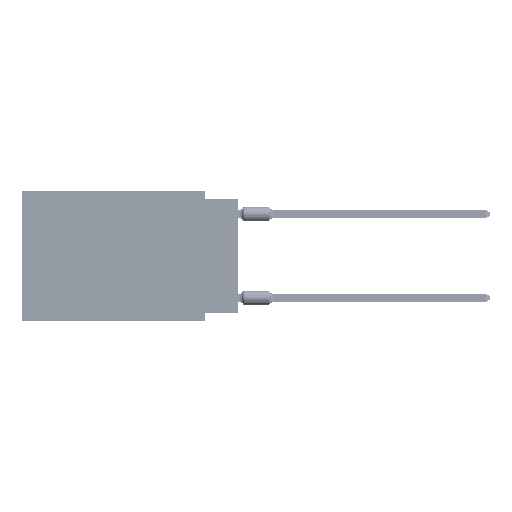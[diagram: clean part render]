
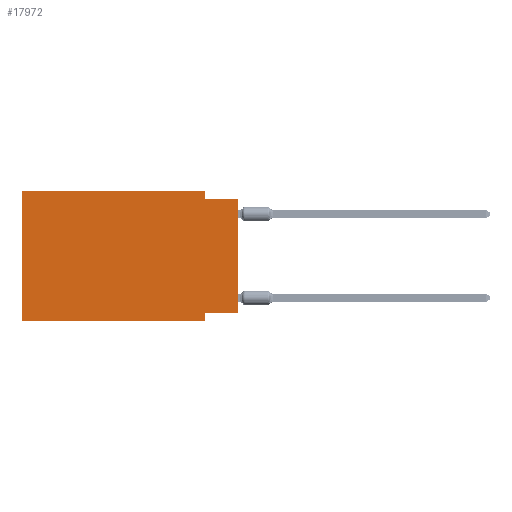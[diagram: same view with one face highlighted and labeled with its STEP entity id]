
A CAD part, left-side view. The second image highlights one B-rep face of the part: STEP entity #17972.
In plain terms, the highlighted planar face has unit normal (-1, 0, 0).
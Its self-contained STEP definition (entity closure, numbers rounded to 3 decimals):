
#256 = CARTESIAN_POINT ( 'NONE',  ( 0., 16.383, 0. ) ) ;
#1149 = VECTOR ( 'NONE', #34853, 1000. ) ;
#2446 = DIRECTION ( 'NONE',  ( 0., 0., -1. ) ) ;
#3097 = FACE_OUTER_BOUND ( 'NONE', #40333, .T. ) ;
#5128 = ORIENTED_EDGE ( 'NONE', *, *, #46602, .F. ) ;
#6071 = VECTOR ( 'NONE', #60997, 1000. ) ;
#8288 = CARTESIAN_POINT ( 'NONE',  ( 0., 2.54, -9.906 ) ) ;
#8918 = EDGE_CURVE ( 'NONE', #62883, #73409, #58326, .T. ) ;
#10476 = DIRECTION ( 'NONE',  ( 0., -1., 0. ) ) ;
#10887 = VECTOR ( 'NONE', #33631, 1000. ) ;
#12662 = VECTOR ( 'NONE', #24476, 1000. ) ;
#12917 = VERTEX_POINT ( 'NONE', #16087 ) ;
#12929 = CARTESIAN_POINT ( 'NONE',  ( 0., 16.383, -9.906 ) ) ;
#14081 = LINE ( 'NONE', #31740, #12662 ) ;
#14102 = CARTESIAN_POINT ( 'NONE',  ( 0., 0., -0.635 ) ) ;
#16087 = CARTESIAN_POINT ( 'NONE',  ( 0., 2.54, -9.906 ) ) ;
#16154 = ORIENTED_EDGE ( 'NONE', *, *, #8918, .F. ) ;
#16762 = EDGE_CURVE ( 'NONE', #73409, #66488, #39295, .T. ) ;
#17756 = CARTESIAN_POINT ( 'NONE',  ( 0., 2.54, -9.271 ) ) ;
#17972 = ADVANCED_FACE ( 'NONE', ( #3097 ), #67305, .F. ) ;
#20250 = CARTESIAN_POINT ( 'NONE',  ( 0., 0., -0.635 ) ) ;
#22064 = CARTESIAN_POINT ( 'NONE',  ( 0., 2.54, 0. ) ) ;
#22687 = VERTEX_POINT ( 'NONE', #72354 ) ;
#24476 = DIRECTION ( 'NONE',  ( 0., 1., 0. ) ) ;
#24966 = AXIS2_PLACEMENT_3D ( 'NONE', #61535, #26523, #49994 ) ;
#25537 = ORIENTED_EDGE ( 'NONE', *, *, #62979, .F. ) ;
#25587 = DIRECTION ( 'NONE',  ( 0., -1., 0. ) ) ;
#26523 = DIRECTION ( 'NONE',  ( 1., 0., 0. ) ) ;
#28707 = VECTOR ( 'NONE', #31718, 1000. ) ;
#31718 = DIRECTION ( 'NONE',  ( 0., 0., -1. ) ) ;
#31740 = CARTESIAN_POINT ( 'NONE',  ( 0., 0., -9.271 ) ) ;
#32106 = CARTESIAN_POINT ( 'NONE',  ( 0., 0., 0. ) ) ;
#33631 = DIRECTION ( 'NONE',  ( 0., 0., 1. ) ) ;
#34049 = VECTOR ( 'NONE', #2446, 1000. ) ;
#34853 = DIRECTION ( 'NONE',  ( 0., 0., 1. ) ) ;
#35749 = VECTOR ( 'NONE', #25587, 1000. ) ;
#39295 = LINE ( 'NONE', #63151, #54275 ) ;
#40333 = EDGE_LOOP ( 'NONE', ( #46205, #74469, #5128, #51011, #16154, #42727, #25537, #71932 ) ) ;
#42505 = EDGE_CURVE ( 'NONE', #55070, #52070, #14081, .T. ) ;
#42727 = ORIENTED_EDGE ( 'NONE', *, *, #53015, .T. ) ;
#43303 = LINE ( 'NONE', #14102, #6071 ) ;
#46205 = ORIENTED_EDGE ( 'NONE', *, *, #50160, .T. ) ;
#46602 = EDGE_CURVE ( 'NONE', #66488, #22687, #60524, .T. ) ;
#49994 = DIRECTION ( 'NONE',  ( 0., 0., -1. ) ) ;
#50160 = EDGE_CURVE ( 'NONE', #55070, #70047, #68257, .T. ) ;
#51011 = ORIENTED_EDGE ( 'NONE', *, *, #16762, .F. ) ;
#52070 = VERTEX_POINT ( 'NONE', #17756 ) ;
#53015 = EDGE_CURVE ( 'NONE', #62883, #12917, #66740, .T. ) ;
#53994 = CARTESIAN_POINT ( 'NONE',  ( 0., 2.54, 0. ) ) ;
#54275 = VECTOR ( 'NONE', #10476, 1000. ) ;
#55070 = VERTEX_POINT ( 'NONE', #61848 ) ;
#58326 = LINE ( 'NONE', #256, #1149 ) ;
#60524 = LINE ( 'NONE', #53994, #34049 ) ;
#60954 = LINE ( 'NONE', #8288, #28707 ) ;
#60997 = DIRECTION ( 'NONE',  ( 0., -1., 0. ) ) ;
#61535 = CARTESIAN_POINT ( 'NONE',  ( 0., 16.383, 0. ) ) ;
#61848 = CARTESIAN_POINT ( 'NONE',  ( 0., 0., -9.271 ) ) ;
#62883 = VERTEX_POINT ( 'NONE', #12929 ) ;
#62979 = EDGE_CURVE ( 'NONE', #52070, #12917, #60954, .T. ) ;
#63151 = CARTESIAN_POINT ( 'NONE',  ( 0., 16.383, 0. ) ) ;
#66488 = VERTEX_POINT ( 'NONE', #22064 ) ;
#66631 = CARTESIAN_POINT ( 'NONE',  ( 0., 16.383, 0. ) ) ;
#66740 = LINE ( 'NONE', #72902, #35749 ) ;
#67305 = PLANE ( 'NONE',  #24966 ) ;
#68257 = LINE ( 'NONE', #32106, #10887 ) ;
#70047 = VERTEX_POINT ( 'NONE', #20250 ) ;
#70083 = EDGE_CURVE ( 'NONE', #22687, #70047, #43303, .T. ) ;
#71932 = ORIENTED_EDGE ( 'NONE', *, *, #42505, .F. ) ;
#72354 = CARTESIAN_POINT ( 'NONE',  ( 0., 2.54, -0.635 ) ) ;
#72902 = CARTESIAN_POINT ( 'NONE',  ( 0., 16.383, -9.906 ) ) ;
#73409 = VERTEX_POINT ( 'NONE', #66631 ) ;
#74469 = ORIENTED_EDGE ( 'NONE', *, *, #70083, .F. ) ;
